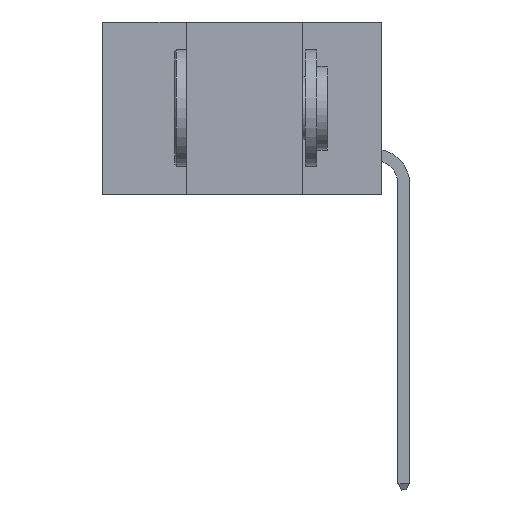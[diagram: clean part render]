
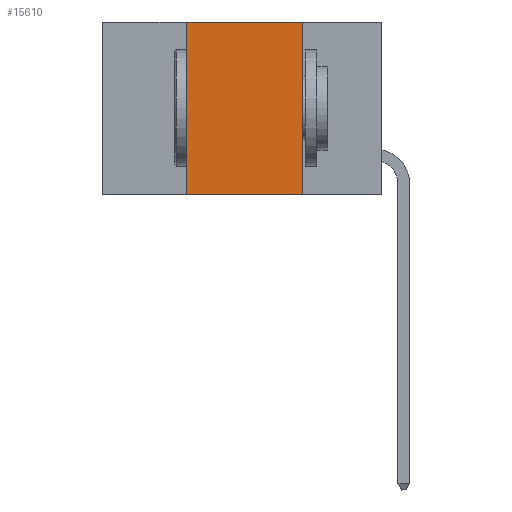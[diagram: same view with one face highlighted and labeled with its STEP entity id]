
A CAD part, left-side view. The second image highlights one B-rep face of the part: STEP entity #15610.
In plain terms, the highlighted planar face has unit normal (-1, 0, 0).
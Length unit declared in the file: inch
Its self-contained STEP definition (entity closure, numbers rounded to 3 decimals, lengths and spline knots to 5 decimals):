
#274 = DIRECTION ( 'NONE',  ( 0., -1., 0. ) ) ;
#496 = DIRECTION ( 'NONE',  ( 0., -1., 0. ) ) ;
#892 = LINE ( 'NONE', #7316, #25816 ) ;
#1024 = CARTESIAN_POINT ( 'NONE',  ( 0., 0.42, 0. ) ) ;
#1281 = LINE ( 'NONE', #11546, #12625 ) ;
#1315 = LINE ( 'NONE', #17029, #18367 ) ;
#7152 = DIRECTION ( 'NONE',  ( 0., 0., -1. ) ) ;
#7316 = CARTESIAN_POINT ( 'NONE',  ( 0., 0.6, -0.37 ) ) ;
#7415 = CARTESIAN_POINT ( 'NONE',  ( 0., 0.17, -0.37 ) ) ;
#8466 = VERTEX_POINT ( 'NONE', #7415 ) ;
#8973 = ORIENTED_EDGE ( 'NONE', *, *, #29024, .F. ) ;
#10922 = VERTEX_POINT ( 'NONE', #1024 ) ;
#11178 = VECTOR ( 'NONE', #274, 39.37008 ) ;
#11546 = CARTESIAN_POINT ( 'NONE',  ( 0., 0.42, 0. ) ) ;
#11739 = DIRECTION ( 'NONE',  ( 0., 0., 1. ) ) ;
#12088 = EDGE_CURVE ( 'NONE', #24302, #8466, #892, .T. ) ;
#12625 = VECTOR ( 'NONE', #11739, 39.37008 ) ;
#12794 = PLANE ( 'NONE',  #20221 ) ;
#13314 = ORIENTED_EDGE ( 'NONE', *, *, #28630, .F. ) ;
#15610 = ADVANCED_FACE ( 'NONE', ( #28253 ), #12794, .F. ) ;
#17029 = CARTESIAN_POINT ( 'NONE',  ( 0., 0.17, 0. ) ) ;
#17088 = CARTESIAN_POINT ( 'NONE',  ( 0., 0.6, 0. ) ) ;
#17603 = VERTEX_POINT ( 'NONE', #25105 ) ;
#17661 = DIRECTION ( 'NONE',  ( 1., 0., 0. ) ) ;
#18367 = VECTOR ( 'NONE', #7152, 39.37008 ) ;
#19099 = LINE ( 'NONE', #17088, #11178 ) ;
#19162 = EDGE_CURVE ( 'NONE', #10922, #17603, #19099, .T. ) ;
#19942 = CARTESIAN_POINT ( 'NONE',  ( 0., 0.6, 0. ) ) ;
#20221 = AXIS2_PLACEMENT_3D ( 'NONE', #19942, #17661, #22355 ) ;
#20605 = EDGE_LOOP ( 'NONE', ( #13314, #27658, #8973, #30254 ) ) ;
#22355 = DIRECTION ( 'NONE',  ( 0., 0., -1. ) ) ;
#24302 = VERTEX_POINT ( 'NONE', #29281 ) ;
#25105 = CARTESIAN_POINT ( 'NONE',  ( 0., 0.17, 0. ) ) ;
#25816 = VECTOR ( 'NONE', #496, 39.37008 ) ;
#27658 = ORIENTED_EDGE ( 'NONE', *, *, #19162, .F. ) ;
#28253 = FACE_OUTER_BOUND ( 'NONE', #20605, .T. ) ;
#28630 = EDGE_CURVE ( 'NONE', #17603, #8466, #1315, .T. ) ;
#29024 = EDGE_CURVE ( 'NONE', #24302, #10922, #1281, .T. ) ;
#29281 = CARTESIAN_POINT ( 'NONE',  ( 0., 0.42, -0.37 ) ) ;
#30254 = ORIENTED_EDGE ( 'NONE', *, *, #12088, .T. ) ;
